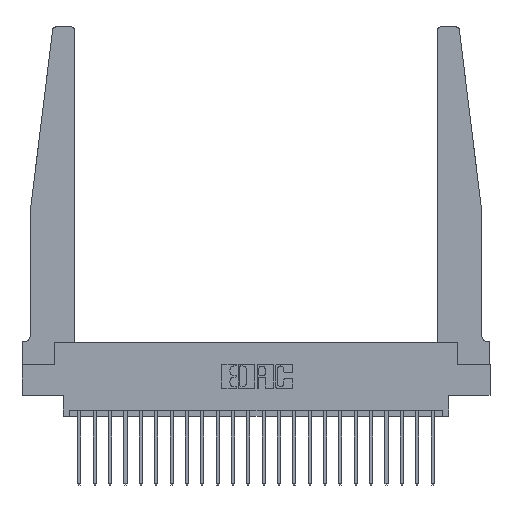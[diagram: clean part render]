
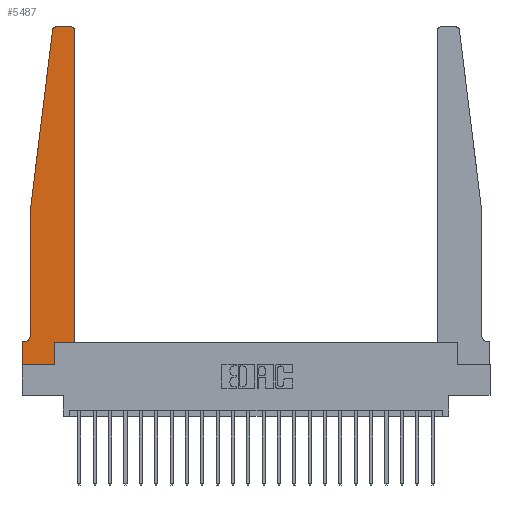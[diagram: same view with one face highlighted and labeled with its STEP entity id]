
A CAD part, top view. The second image highlights one B-rep face of the part: STEP entity #5487.
In plain terms, the highlighted planar face has unit normal (0, 0, 1).
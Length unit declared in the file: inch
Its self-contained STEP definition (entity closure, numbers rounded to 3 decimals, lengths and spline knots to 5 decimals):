
#6 = DIRECTION ( 'NONE',  ( 0., 0., 1. ) ) ;
#174 = CARTESIAN_POINT ( 'NONE',  ( 0.395, 2.72, 0.37 ) ) ;
#330 = DIRECTION ( 'NONE',  ( 0., -1., 0. ) ) ;
#940 = EDGE_CURVE ( 'NONE', #16674, #17046, #2049, .T. ) ;
#996 = ORIENTED_EDGE ( 'NONE', *, *, #5363, .T. ) ;
#1132 = VECTOR ( 'NONE', #15821, 39.37008 ) ;
#1259 = ORIENTED_EDGE ( 'NONE', *, *, #5810, .T. ) ;
#1404 = DIRECTION ( 'NONE',  ( -1., 0., 0. ) ) ;
#1757 = CARTESIAN_POINT ( 'NONE',  ( 0.065, 1.25, 0.37 ) ) ;
#1932 = DIRECTION ( 'NONE',  ( 1., 0., 0. ) ) ;
#2038 = DIRECTION ( 'NONE',  ( 0., 1., 0. ) ) ;
#2049 = LINE ( 'NONE', #22340, #6199 ) ;
#2056 = VECTOR ( 'NONE', #2038, 39.37008 ) ;
#2635 = ORIENTED_EDGE ( 'NONE', *, *, #17736, .T. ) ;
#2770 = DIRECTION ( 'NONE',  ( 0., 0., 1. ) ) ;
#2794 = CARTESIAN_POINT ( 'NONE',  ( 0., 0., 0.37 ) ) ;
#3213 = VERTEX_POINT ( 'NONE', #11999 ) ;
#3423 = EDGE_CURVE ( 'NONE', #3213, #20346, #17822, .T. ) ;
#3628 = FACE_OUTER_BOUND ( 'NONE', #17407, .T. ) ;
#3825 = CARTESIAN_POINT ( 'NONE',  ( 0.425, 0.18, 0.37 ) ) ;
#4140 = CARTESIAN_POINT ( 'NONE',  ( 0., 0., 0.37 ) ) ;
#4445 = DIRECTION ( 'NONE',  ( 0., 0., -1. ) ) ;
#4571 = ORIENTED_EDGE ( 'NONE', *, *, #14128, .T. ) ;
#4616 = EDGE_CURVE ( 'NONE', #17046, #12712, #14950, .T. ) ;
#4800 = CARTESIAN_POINT ( 'NONE',  ( 0.015, 0.1875, 0.37 ) ) ;
#4837 = VERTEX_POINT ( 'NONE', #8514 ) ;
#4953 = CARTESIAN_POINT ( 'NONE',  ( 0.27653, 2.75, 0.37 ) ) ;
#5223 = CARTESIAN_POINT ( 'NONE',  ( 0.425, 0.18, 0.37 ) ) ;
#5363 = EDGE_CURVE ( 'NONE', #17915, #21960, #16385, .T. ) ;
#5487 = ADVANCED_FACE ( 'NONE', ( #3628 ), #19520, .T. ) ;
#5810 = EDGE_CURVE ( 'NONE', #15851, #4837, #13302, .T. ) ;
#5828 = LINE ( 'NONE', #5223, #1132 ) ;
#6103 = EDGE_CURVE ( 'NONE', #4837, #16674, #7184, .T. ) ;
#6199 = VECTOR ( 'NONE', #22265, 39.37008 ) ;
#6635 = VECTOR ( 'NONE', #15918, 39.37008 ) ;
#6893 = LINE ( 'NONE', #2794, #21131 ) ;
#7021 = CARTESIAN_POINT ( 'NONE',  ( 0.2605, 0.18, 0.37 ) ) ;
#7047 = ORIENTED_EDGE ( 'NONE', *, *, #6103, .T. ) ;
#7184 = LINE ( 'NONE', #1757, #6635 ) ;
#7460 = CARTESIAN_POINT ( 'NONE',  ( 0.395, 2.75, 0.37 ) ) ;
#8129 = ORIENTED_EDGE ( 'NONE', *, *, #940, .T. ) ;
#8514 = CARTESIAN_POINT ( 'NONE',  ( 0.24675, 2.72367, 0.37 ) ) ;
#8525 = LINE ( 'NONE', #14938, #21675 ) ;
#8786 = CARTESIAN_POINT ( 'NONE',  ( 0.065, 0.2375, 0.37 ) ) ;
#9257 = ORIENTED_EDGE ( 'NONE', *, *, #11302, .T. ) ;
#9384 = VERTEX_POINT ( 'NONE', #12928 ) ;
#10594 = CARTESIAN_POINT ( 'NONE',  ( 0., 0.1875, 0.37 ) ) ;
#10675 = VERTEX_POINT ( 'NONE', #4140 ) ;
#10720 = AXIS2_PLACEMENT_3D ( 'NONE', #10594, #6, #12381 ) ;
#11160 = VECTOR ( 'NONE', #330, 39.37008 ) ;
#11302 = EDGE_CURVE ( 'NONE', #9384, #10675, #16439, .T. ) ;
#11999 = CARTESIAN_POINT ( 'NONE',  ( 0.425, 2.72, 0.37 ) ) ;
#12055 = ORIENTED_EDGE ( 'NONE', *, *, #3423, .T. ) ;
#12082 = CARTESIAN_POINT ( 'NONE',  ( 0.2605, 0.18, 0.37 ) ) ;
#12381 = DIRECTION ( 'NONE',  ( 1., 0., 0. ) ) ;
#12529 = DIRECTION ( 'NONE',  ( 0., 0., 1. ) ) ;
#12656 = AXIS2_PLACEMENT_3D ( 'NONE', #13366, #2770, #15163 ) ;
#12712 = VERTEX_POINT ( 'NONE', #4800 ) ;
#12925 = CARTESIAN_POINT ( 'NONE',  ( 0.065, 1.25, 0.37 ) ) ;
#12928 = CARTESIAN_POINT ( 'NONE',  ( 0., 0.1875, 0.37 ) ) ;
#13302 = CIRCLE ( 'NONE', #12656, 0.03 ) ;
#13366 = CARTESIAN_POINT ( 'NONE',  ( 0.27653, 2.72, 0.37 ) ) ;
#13429 = ORIENTED_EDGE ( 'NONE', *, *, #4616, .T. ) ;
#13798 = CARTESIAN_POINT ( 'NONE',  ( 0.065, 0.1875, 0.37 ) ) ;
#13872 = DIRECTION ( 'NONE',  ( 0., 1., 0. ) ) ;
#13989 = EDGE_CURVE ( 'NONE', #10675, #17915, #6893, .T. ) ;
#14039 = VERTEX_POINT ( 'NONE', #17076 ) ;
#14128 = EDGE_CURVE ( 'NONE', #12712, #9384, #18338, .T. ) ;
#14437 = EDGE_CURVE ( 'NONE', #20346, #15851, #8525, .T. ) ;
#14563 = ORIENTED_EDGE ( 'NONE', *, *, #13989, .T. ) ;
#14938 = CARTESIAN_POINT ( 'NONE',  ( 0.25, 2.75, 0.37 ) ) ;
#14950 = CIRCLE ( 'NONE', #22825, 0.05 ) ;
#15057 = CARTESIAN_POINT ( 'NONE',  ( 0.015, 0.2375, 0.37 ) ) ;
#15163 = DIRECTION ( 'NONE',  ( 1., 0., 0. ) ) ;
#15190 = DIRECTION ( 'NONE',  ( 1., 0., 0. ) ) ;
#15271 = VECTOR ( 'NONE', #13872, 39.37008 ) ;
#15821 = DIRECTION ( 'NONE',  ( 1., 0., 0. ) ) ;
#15851 = VERTEX_POINT ( 'NONE', #4953 ) ;
#15918 = DIRECTION ( 'NONE',  ( -0.122, -0.992, 0. ) ) ;
#16385 = LINE ( 'NONE', #12082, #15271 ) ;
#16439 = LINE ( 'NONE', #18111, #11160 ) ;
#16674 = VERTEX_POINT ( 'NONE', #12925 ) ;
#16862 = DIRECTION ( 'NONE',  ( -1., 0., 0. ) ) ;
#17046 = VERTEX_POINT ( 'NONE', #8786 ) ;
#17076 = CARTESIAN_POINT ( 'NONE',  ( 0.425, 0.18, 0.37 ) ) ;
#17407 = EDGE_LOOP ( 'NONE', ( #19614, #1259, #7047, #8129, #13429, #4571, #9257, #14563, #996, #19909, #2635, #12055 ) ) ;
#17736 = EDGE_CURVE ( 'NONE', #14039, #3213, #20984, .T. ) ;
#17822 = CIRCLE ( 'NONE', #19841, 0.03 ) ;
#17915 = VERTEX_POINT ( 'NONE', #20631 ) ;
#18111 = CARTESIAN_POINT ( 'NONE',  ( 0., 0., 0.37 ) ) ;
#18338 = LINE ( 'NONE', #13798, #19460 ) ;
#18565 = DIRECTION ( 'NONE',  ( -1., 0., 0. ) ) ;
#19460 = VECTOR ( 'NONE', #1404, 39.37008 ) ;
#19520 = PLANE ( 'NONE',  #10720 ) ;
#19614 = ORIENTED_EDGE ( 'NONE', *, *, #14437, .T. ) ;
#19841 = AXIS2_PLACEMENT_3D ( 'NONE', #174, #12529, #1932 ) ;
#19909 = ORIENTED_EDGE ( 'NONE', *, *, #22515, .T. ) ;
#20346 = VERTEX_POINT ( 'NONE', #7460 ) ;
#20631 = CARTESIAN_POINT ( 'NONE',  ( 0.2605, 0., 0.37 ) ) ;
#20984 = LINE ( 'NONE', #3825, #2056 ) ;
#21131 = VECTOR ( 'NONE', #15190, 39.37008 ) ;
#21675 = VECTOR ( 'NONE', #18565, 39.37008 ) ;
#21960 = VERTEX_POINT ( 'NONE', #7021 ) ;
#22265 = DIRECTION ( 'NONE',  ( 0., -1., 0. ) ) ;
#22340 = CARTESIAN_POINT ( 'NONE',  ( 0.065, 1.25, 0.37 ) ) ;
#22515 = EDGE_CURVE ( 'NONE', #21960, #14039, #5828, .T. ) ;
#22825 = AXIS2_PLACEMENT_3D ( 'NONE', #15057, #4445, #16862 ) ;
